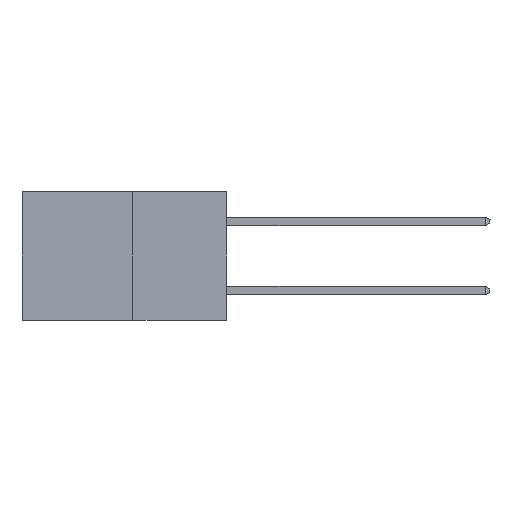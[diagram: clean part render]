
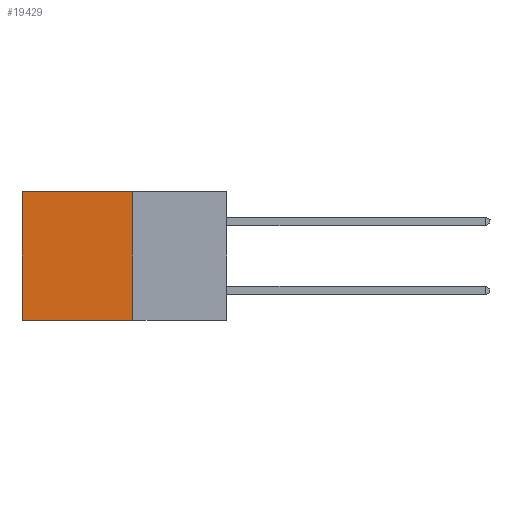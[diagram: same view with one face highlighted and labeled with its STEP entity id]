
A CAD part, left-side view. The second image highlights one B-rep face of the part: STEP entity #19429.
In plain terms, the highlighted planar face has unit normal (-1, 0, 0).
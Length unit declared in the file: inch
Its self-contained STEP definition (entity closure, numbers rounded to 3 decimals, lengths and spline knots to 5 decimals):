
#19 = EDGE_CURVE ( 'NONE', #15659, #4658, #5592, .T. ) ;
#482 = FACE_OUTER_BOUND ( 'NONE', #3077, .T. ) ;
#715 = VECTOR ( 'NONE', #12465, 39.37008 ) ;
#1810 = VERTEX_POINT ( 'NONE', #12695 ) ;
#1855 = LINE ( 'NONE', #5439, #6260 ) ;
#2879 = DIRECTION ( 'NONE',  ( 0., 0., -1. ) ) ;
#2891 = PLANE ( 'NONE',  #4930 ) ;
#2989 = CARTESIAN_POINT ( 'NONE',  ( 0.277, 0.59, -0.37 ) ) ;
#3077 = EDGE_LOOP ( 'NONE', ( #9427, #13696, #14885, #6971 ) ) ;
#4658 = VERTEX_POINT ( 'NONE', #14110 ) ;
#4930 = AXIS2_PLACEMENT_3D ( 'NONE', #6247, #16930, #7820 ) ;
#5439 = CARTESIAN_POINT ( 'NONE',  ( 0.277, 0.27, 0. ) ) ;
#5592 = LINE ( 'NONE', #19534, #715 ) ;
#6232 = EDGE_CURVE ( 'NONE', #1810, #11721, #15021, .T. ) ;
#6247 = CARTESIAN_POINT ( 'NONE',  ( 0.277, 0.27, -0.37 ) ) ;
#6260 = VECTOR ( 'NONE', #13242, 39.37008 ) ;
#6971 = ORIENTED_EDGE ( 'NONE', *, *, #10831, .T. ) ;
#7502 = CARTESIAN_POINT ( 'NONE',  ( 0.277, 0.27, -0.37 ) ) ;
#7820 = DIRECTION ( 'NONE',  ( 0., 0., -1. ) ) ;
#9427 = ORIENTED_EDGE ( 'NONE', *, *, #6232, .T. ) ;
#9679 = CARTESIAN_POINT ( 'NONE',  ( 0.277, 0.27, 0. ) ) ;
#10831 = EDGE_CURVE ( 'NONE', #15659, #1810, #1855, .T. ) ;
#11016 = VECTOR ( 'NONE', #2879, 39.37008 ) ;
#11721 = VERTEX_POINT ( 'NONE', #16708 ) ;
#12465 = DIRECTION ( 'NONE',  ( 0., 0., -1. ) ) ;
#12500 = LINE ( 'NONE', #7502, #19984 ) ;
#12695 = CARTESIAN_POINT ( 'NONE',  ( 0.277, 0.59, 0. ) ) ;
#13242 = DIRECTION ( 'NONE',  ( 0., 1., 0. ) ) ;
#13696 = ORIENTED_EDGE ( 'NONE', *, *, #16058, .F. ) ;
#14110 = CARTESIAN_POINT ( 'NONE',  ( 0.277, 0.27, -0.37 ) ) ;
#14885 = ORIENTED_EDGE ( 'NONE', *, *, #19, .F. ) ;
#15021 = LINE ( 'NONE', #2989, #11016 ) ;
#15659 = VERTEX_POINT ( 'NONE', #9679 ) ;
#16058 = EDGE_CURVE ( 'NONE', #4658, #11721, #12500, .T. ) ;
#16708 = CARTESIAN_POINT ( 'NONE',  ( 0.277, 0.59, -0.37 ) ) ;
#16930 = DIRECTION ( 'NONE',  ( 1., 0., 0. ) ) ;
#18119 = DIRECTION ( 'NONE',  ( 0., 1., 0. ) ) ;
#19429 = ADVANCED_FACE ( 'NONE', ( #482 ), #2891, .F. ) ;
#19534 = CARTESIAN_POINT ( 'NONE',  ( 0.277, 0.27, -0.37 ) ) ;
#19984 = VECTOR ( 'NONE', #18119, 39.37008 ) ;
